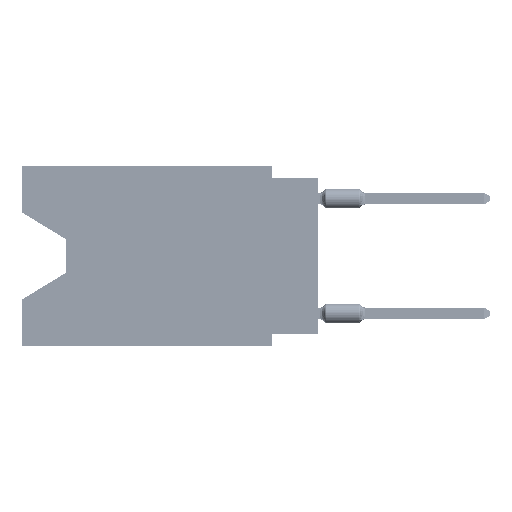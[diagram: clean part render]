
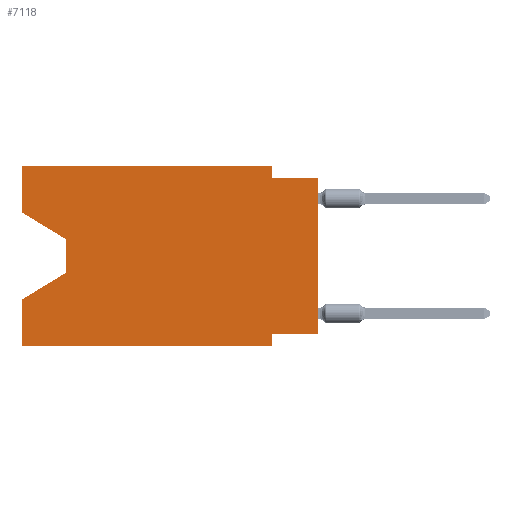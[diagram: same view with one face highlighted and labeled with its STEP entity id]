
A CAD part, left-side view. The second image highlights one B-rep face of the part: STEP entity #7118.
In plain terms, the highlighted planar face has unit normal (-1, 0, 0).
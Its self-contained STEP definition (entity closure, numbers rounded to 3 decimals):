
#604 = DIRECTION ( 'NONE',  ( 1., 0., 0. ) ) ;
#2841 = DIRECTION ( 'NONE',  ( 0., 0.855, -0.519 ) ) ;
#3817 = VECTOR ( 'NONE', #48825, 1000. ) ;
#3990 = EDGE_CURVE ( 'NONE', #28335, #47878, #5574, .T. ) ;
#5574 = LINE ( 'NONE', #36810, #25514 ) ;
#5798 = VECTOR ( 'NONE', #20451, 1000. ) ;
#6386 = CARTESIAN_POINT ( 'NONE',  ( 0., 16.383, -9.906 ) ) ;
#6600 = DIRECTION ( 'NONE',  ( 0., 0., -1. ) ) ;
#7118 = ADVANCED_FACE ( 'NONE', ( #7861 ), #65553, .F. ) ;
#7306 = ORIENTED_EDGE ( 'NONE', *, *, #3990, .F. ) ;
#7576 = LINE ( 'NONE', #54122, #33588 ) ;
#7861 = FACE_OUTER_BOUND ( 'NONE', #77979, .T. ) ;
#7916 = ORIENTED_EDGE ( 'NONE', *, *, #62609, .F. ) ;
#8903 = CARTESIAN_POINT ( 'NONE',  ( 0., 16.383, 0. ) ) ;
#9063 = CARTESIAN_POINT ( 'NONE',  ( 0., 16.383, 0. ) ) ;
#10115 = CARTESIAN_POINT ( 'NONE',  ( 0., 13.97, -5.893 ) ) ;
#11729 = CARTESIAN_POINT ( 'NONE',  ( 0., 13.97, -4.013 ) ) ;
#12670 = LINE ( 'NONE', #18661, #84363 ) ;
#12728 = VERTEX_POINT ( 'NONE', #28929 ) ;
#14899 = LINE ( 'NONE', #8903, #5798 ) ;
#15207 = VERTEX_POINT ( 'NONE', #41870 ) ;
#17474 = VERTEX_POINT ( 'NONE', #78360 ) ;
#18661 = CARTESIAN_POINT ( 'NONE',  ( 0., 16.383, -2.546 ) ) ;
#20451 = DIRECTION ( 'NONE',  ( 0., 0., 1. ) ) ;
#21405 = VERTEX_POINT ( 'NONE', #48975 ) ;
#21514 = LINE ( 'NONE', #49250, #3817 ) ;
#22791 = ORIENTED_EDGE ( 'NONE', *, *, #24819, .F. ) ;
#23137 = VERTEX_POINT ( 'NONE', #48867 ) ;
#23296 = LINE ( 'NONE', #11729, #77868 ) ;
#23578 = LINE ( 'NONE', #9063, #40685 ) ;
#24606 = CARTESIAN_POINT ( 'NONE',  ( 0., 2.54, -9.906 ) ) ;
#24819 = EDGE_CURVE ( 'NONE', #15207, #21405, #23578, .T. ) ;
#25514 = VECTOR ( 'NONE', #30837, 1000. ) ;
#27269 = AXIS2_PLACEMENT_3D ( 'NONE', #58710, #604, #6600 ) ;
#28335 = VERTEX_POINT ( 'NONE', #56412 ) ;
#28400 = CARTESIAN_POINT ( 'NONE',  ( 0., 13.97, -4.013 ) ) ;
#28929 = CARTESIAN_POINT ( 'NONE',  ( 0., 2.54, -9.906 ) ) ;
#29085 = VERTEX_POINT ( 'NONE', #73756 ) ;
#29227 = EDGE_CURVE ( 'NONE', #29085, #12728, #30601, .T. ) ;
#29548 = VERTEX_POINT ( 'NONE', #68403 ) ;
#29615 = EDGE_CURVE ( 'NONE', #23137, #28335, #14899, .T. ) ;
#30542 = DIRECTION ( 'NONE',  ( 0., 0., -1. ) ) ;
#30601 = LINE ( 'NONE', #24606, #54842 ) ;
#30751 = CARTESIAN_POINT ( 'NONE',  ( 0., 2.54, 0. ) ) ;
#30837 = DIRECTION ( 'NONE',  ( 0., -1., 0. ) ) ;
#31872 = ORIENTED_EDGE ( 'NONE', *, *, #45070, .T. ) ;
#33588 = VECTOR ( 'NONE', #33643, 1000. ) ;
#33643 = DIRECTION ( 'NONE',  ( 0., 1., 0. ) ) ;
#35005 = CARTESIAN_POINT ( 'NONE',  ( 0., 0., -0.635 ) ) ;
#36458 = EDGE_CURVE ( 'NONE', #29548, #66224, #21514, .T. ) ;
#36810 = CARTESIAN_POINT ( 'NONE',  ( 0., 16.383, 0. ) ) ;
#38306 = EDGE_CURVE ( 'NONE', #23137, #71274, #12670, .T. ) ;
#39287 = ORIENTED_EDGE ( 'NONE', *, *, #38306, .T. ) ;
#39633 = ORIENTED_EDGE ( 'NONE', *, *, #68068, .F. ) ;
#40498 = LINE ( 'NONE', #53321, #60072 ) ;
#40685 = VECTOR ( 'NONE', #75252, 1000. ) ;
#40733 = EDGE_CURVE ( 'NONE', #65139, #66224, #40498, .T. ) ;
#41870 = CARTESIAN_POINT ( 'NONE',  ( 0., 16.383, -9.906 ) ) ;
#45070 = EDGE_CURVE ( 'NONE', #15207, #12728, #77748, .T. ) ;
#45957 = LINE ( 'NONE', #30751, #83241 ) ;
#46374 = DIRECTION ( 'NONE',  ( 0., -0.855, -0.519 ) ) ;
#46507 = DIRECTION ( 'NONE',  ( 0., -1., 0. ) ) ;
#47114 = ORIENTED_EDGE ( 'NONE', *, *, #29227, .F. ) ;
#47854 = CARTESIAN_POINT ( 'NONE',  ( 0., 2.54, -0.635 ) ) ;
#47878 = VERTEX_POINT ( 'NONE', #73200 ) ;
#48825 = DIRECTION ( 'NONE',  ( 0., 0., 1. ) ) ;
#48867 = CARTESIAN_POINT ( 'NONE',  ( 0., 16.383, -2.546 ) ) ;
#48975 = CARTESIAN_POINT ( 'NONE',  ( 0., 16.383, -7.36 ) ) ;
#49250 = CARTESIAN_POINT ( 'NONE',  ( 0., 0., 0. ) ) ;
#49962 = DIRECTION ( 'NONE',  ( 0., 0., -1. ) ) ;
#50358 = VECTOR ( 'NONE', #2841, 1000. ) ;
#52067 = EDGE_CURVE ( 'NONE', #17474, #21405, #68626, .T. ) ;
#53321 = CARTESIAN_POINT ( 'NONE',  ( 0., 0., -0.635 ) ) ;
#54122 = CARTESIAN_POINT ( 'NONE',  ( 0., 0., -9.271 ) ) ;
#54458 = ORIENTED_EDGE ( 'NONE', *, *, #68433, .T. ) ;
#54842 = VECTOR ( 'NONE', #63460, 1000. ) ;
#56412 = CARTESIAN_POINT ( 'NONE',  ( 0., 16.383, 0. ) ) ;
#56510 = VECTOR ( 'NONE', #71735, 1000. ) ;
#58293 = ORIENTED_EDGE ( 'NONE', *, *, #29615, .F. ) ;
#58710 = CARTESIAN_POINT ( 'NONE',  ( 0., 16.383, 0. ) ) ;
#60072 = VECTOR ( 'NONE', #46507, 1000. ) ;
#62609 = EDGE_CURVE ( 'NONE', #29548, #29085, #7576, .T. ) ;
#63460 = DIRECTION ( 'NONE',  ( 0., 0., -1. ) ) ;
#65139 = VERTEX_POINT ( 'NONE', #47854 ) ;
#65553 = PLANE ( 'NONE',  #27269 ) ;
#66224 = VERTEX_POINT ( 'NONE', #35005 ) ;
#68068 = EDGE_CURVE ( 'NONE', #47878, #65139, #45957, .T. ) ;
#68341 = ORIENTED_EDGE ( 'NONE', *, *, #36458, .T. ) ;
#68403 = CARTESIAN_POINT ( 'NONE',  ( 0., 0., -9.271 ) ) ;
#68433 = EDGE_CURVE ( 'NONE', #71274, #17474, #23296, .T. ) ;
#68626 = LINE ( 'NONE', #10115, #50358 ) ;
#70126 = ORIENTED_EDGE ( 'NONE', *, *, #40733, .F. ) ;
#71274 = VERTEX_POINT ( 'NONE', #28400 ) ;
#71735 = DIRECTION ( 'NONE',  ( 0., -1., 0. ) ) ;
#73200 = CARTESIAN_POINT ( 'NONE',  ( 0., 2.54, 0. ) ) ;
#73756 = CARTESIAN_POINT ( 'NONE',  ( 0., 2.54, -9.271 ) ) ;
#75252 = DIRECTION ( 'NONE',  ( 0., 0., 1. ) ) ;
#76565 = ORIENTED_EDGE ( 'NONE', *, *, #52067, .T. ) ;
#77748 = LINE ( 'NONE', #6386, #56510 ) ;
#77868 = VECTOR ( 'NONE', #30542, 1000. ) ;
#77979 = EDGE_LOOP ( 'NONE', ( #39287, #54458, #76565, #22791, #31872, #47114, #7916, #68341, #70126, #39633, #7306, #58293 ) ) ;
#78360 = CARTESIAN_POINT ( 'NONE',  ( 0., 13.97, -5.893 ) ) ;
#83241 = VECTOR ( 'NONE', #49962, 1000. ) ;
#84363 = VECTOR ( 'NONE', #46374, 1000. ) ;
